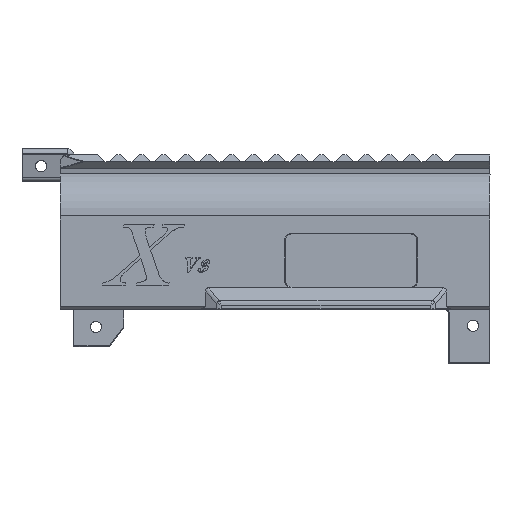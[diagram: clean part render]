
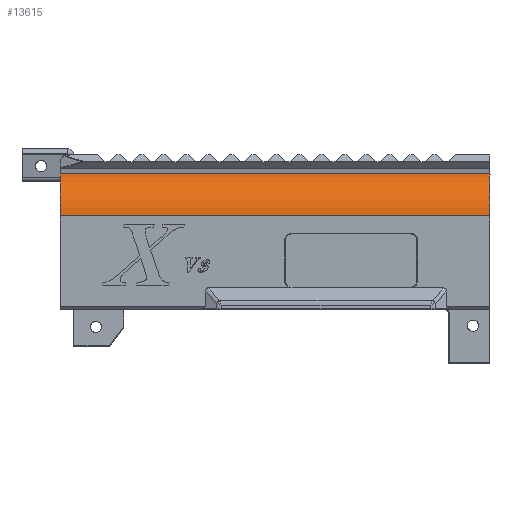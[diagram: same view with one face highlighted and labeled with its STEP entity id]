
A CAD part, top view. The second image highlights one B-rep face of the part: STEP entity #13615.
In plain terms, the highlighted cylindrical face has radius 20.1 mm (diameter 40.2 mm), a partial arc.
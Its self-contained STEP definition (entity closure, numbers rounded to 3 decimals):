
#283 = DIRECTION ( 'NONE',  ( 0., 0., -1. ) ) ;
#1854 = VERTEX_POINT ( 'NONE', #10839 ) ;
#1873 = CARTESIAN_POINT ( 'NONE',  ( 11.578, 47.361, 21.1 ) ) ;
#2029 = AXIS2_PLACEMENT_3D ( 'NONE', #7683, #10094, #3759 ) ;
#2145 = CARTESIAN_POINT ( 'NONE',  ( -20.172, 47.361, 21.1 ) ) ;
#2306 = LINE ( 'NONE', #2145, #7415 ) ;
#3504 = DIRECTION ( 'NONE',  ( 0., 0., -1. ) ) ;
#3759 = DIRECTION ( 'NONE',  ( 0., 0., -1. ) ) ;
#3829 = EDGE_CURVE ( 'NONE', #15540, #6574, #10814, .T. ) ;
#4528 = CARTESIAN_POINT ( 'NONE',  ( -178.804, 65.991, 8.545 ) ) ;
#4793 = EDGE_CURVE ( 'NONE', #15540, #1854, #2306, .T. ) ;
#4911 = ORIENTED_EDGE ( 'NONE', *, *, #10188, .T. ) ;
#5011 = FACE_OUTER_BOUND ( 'NONE', #13918, .T. ) ;
#5098 = CYLINDRICAL_SURFACE ( 'NONE', #2029, 20.1 ) ;
#5766 = DIRECTION ( 'NONE',  ( 1., 0., 0. ) ) ;
#5846 = EDGE_CURVE ( 'NONE', #10476, #1854, #10109, .T. ) ;
#6110 = AXIS2_PLACEMENT_3D ( 'NONE', #7267, #5766, #3504 ) ;
#6210 = VECTOR ( 'NONE', #8300, 1000. ) ;
#6574 = VERTEX_POINT ( 'NONE', #15062 ) ;
#6804 = CARTESIAN_POINT ( 'NONE',  ( 11.578, 47.361, 1. ) ) ;
#7267 = CARTESIAN_POINT ( 'NONE',  ( -178.804, 47.361, 1. ) ) ;
#7415 = VECTOR ( 'NONE', #15068, 1000. ) ;
#7683 = CARTESIAN_POINT ( 'NONE',  ( -20.172, 47.361, 1. ) ) ;
#7893 = AXIS2_PLACEMENT_3D ( 'NONE', #6804, #11969, #283 ) ;
#8300 = DIRECTION ( 'NONE',  ( -1., 0., 0. ) ) ;
#10094 = DIRECTION ( 'NONE',  ( 1., 0., 0. ) ) ;
#10109 = CIRCLE ( 'NONE', #6110, 20.1 ) ;
#10188 = EDGE_CURVE ( 'NONE', #6574, #10476, #10792, .T. ) ;
#10476 = VERTEX_POINT ( 'NONE', #4528 ) ;
#10788 = ORIENTED_EDGE ( 'NONE', *, *, #4793, .F. ) ;
#10792 = LINE ( 'NONE', #14456, #6210 ) ;
#10814 = CIRCLE ( 'NONE', #7893, 20.1 ) ;
#10839 = CARTESIAN_POINT ( 'NONE',  ( -178.804, 47.361, 21.1 ) ) ;
#11969 = DIRECTION ( 'NONE',  ( -1., 0., 0. ) ) ;
#13615 = ADVANCED_FACE ( 'NONE', ( #5011 ), #5098, .T. ) ;
#13714 = ORIENTED_EDGE ( 'NONE', *, *, #5846, .T. ) ;
#13918 = EDGE_LOOP ( 'NONE', ( #16332, #4911, #13714, #10788 ) ) ;
#14456 = CARTESIAN_POINT ( 'NONE',  ( -20.172, 65.991, 8.545 ) ) ;
#15062 = CARTESIAN_POINT ( 'NONE',  ( 11.578, 65.991, 8.545 ) ) ;
#15068 = DIRECTION ( 'NONE',  ( -1., 0., 0. ) ) ;
#15540 = VERTEX_POINT ( 'NONE', #1873 ) ;
#16332 = ORIENTED_EDGE ( 'NONE', *, *, #3829, .T. ) ;
